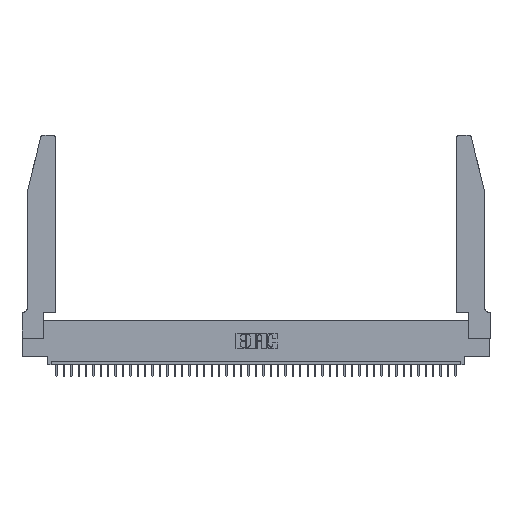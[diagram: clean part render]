
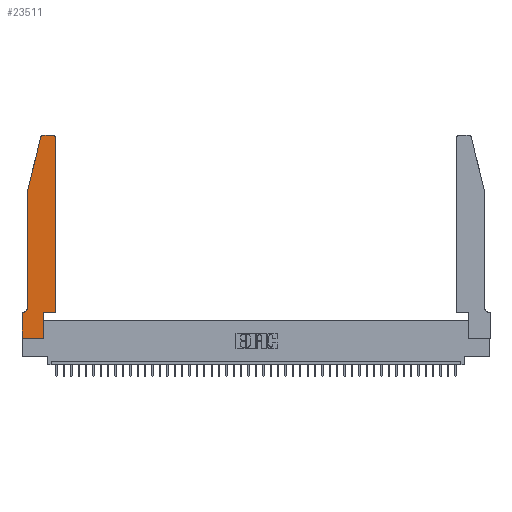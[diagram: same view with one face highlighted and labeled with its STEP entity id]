
A CAD part, top view. The second image highlights one B-rep face of the part: STEP entity #23511.
In plain terms, the highlighted planar face has unit normal (0, 0, 1).
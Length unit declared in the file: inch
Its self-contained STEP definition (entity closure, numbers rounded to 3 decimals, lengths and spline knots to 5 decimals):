
#9 = LINE ( 'NONE', #19868, #17234 ) ;
#221 = EDGE_CURVE ( 'NONE', #9567, #36295, #20676, .T. ) ;
#1085 = CIRCLE ( 'NONE', #24405, 0.07 ) ;
#1886 = DIRECTION ( 'NONE',  ( 0., 1., 0. ) ) ;
#2958 = VECTOR ( 'NONE', #28050, 39.37008 ) ;
#3400 = LINE ( 'NONE', #31642, #19021 ) ;
#4029 = CARTESIAN_POINT ( 'NONE',  ( 0.0755, 2., 0.37 ) ) ;
#4107 = EDGE_LOOP ( 'NONE', ( #40600, #10642, #42172, #23127, #11928, #31680, #28191, #36041, #9734, #17032, #40206, #28281 ) ) ;
#4935 = DIRECTION ( 'NONE',  ( -1., 0., 0. ) ) ;
#5293 = VERTEX_POINT ( 'NONE', #27888 ) ;
#7151 = DIRECTION ( 'NONE',  ( 0., 0., 1. ) ) ;
#7639 = LINE ( 'NONE', #30209, #44311 ) ;
#9567 = VERTEX_POINT ( 'NONE', #40559 ) ;
#9646 = EDGE_CURVE ( 'NONE', #19961, #39414, #7639, .T. ) ;
#9734 = ORIENTED_EDGE ( 'NONE', *, *, #16842, .T. ) ;
#10638 = CARTESIAN_POINT ( 'NONE',  ( 0.2865, 0., 0.37 ) ) ;
#10642 = ORIENTED_EDGE ( 'NONE', *, *, #14025, .T. ) ;
#10894 = EDGE_CURVE ( 'NONE', #28422, #9567, #1085, .T. ) ;
#11406 = FACE_OUTER_BOUND ( 'NONE', #4107, .T. ) ;
#11442 = DIRECTION ( 'NONE',  ( 1., 0., 0. ) ) ;
#11928 = ORIENTED_EDGE ( 'NONE', *, *, #10894, .T. ) ;
#11973 = EDGE_CURVE ( 'NONE', #24701, #5293, #9, .T. ) ;
#12093 = LINE ( 'NONE', #4029, #2958 ) ;
#12349 = LINE ( 'NONE', #12561, #28568 ) ;
#12561 = CARTESIAN_POINT ( 'NONE',  ( 0.2865, 0.35, 0.37 ) ) ;
#12959 = CARTESIAN_POINT ( 'NONE',  ( 0., 0., 0.37 ) ) ;
#13443 = VERTEX_POINT ( 'NONE', #16034 ) ;
#14023 = AXIS2_PLACEMENT_3D ( 'NONE', #44610, #16250, #37972 ) ;
#14025 = EDGE_CURVE ( 'NONE', #13443, #28636, #24495, .T. ) ;
#14664 = VECTOR ( 'NONE', #24942, 39.37008 ) ;
#15070 = CARTESIAN_POINT ( 'NONE',  ( 0.0755, 0.35, 0.37 ) ) ;
#16034 = CARTESIAN_POINT ( 'NONE',  ( 0.284, 2.75, 0.37 ) ) ;
#16250 = DIRECTION ( 'NONE',  ( 0., 0., 1. ) ) ;
#16370 = CARTESIAN_POINT ( 'NONE',  ( 0.0055, 0.42, 0.37 ) ) ;
#16842 = EDGE_CURVE ( 'NONE', #39414, #24701, #12349, .T. ) ;
#17032 = ORIENTED_EDGE ( 'NONE', *, *, #11973, .T. ) ;
#17118 = EDGE_CURVE ( 'NONE', #5293, #40108, #32338, .T. ) ;
#17234 = VECTOR ( 'NONE', #30311, 39.37008 ) ;
#17443 = VECTOR ( 'NONE', #4935, 39.37008 ) ;
#18944 = CARTESIAN_POINT ( 'NONE',  ( 0.0755, 2., 0.37 ) ) ;
#19010 = DIRECTION ( 'NONE',  ( 0., -1., 0. ) ) ;
#19021 = VECTOR ( 'NONE', #34982, 39.37008 ) ;
#19833 = CARTESIAN_POINT ( 'NONE',  ( 0.4205, 2.72, 0.37 ) ) ;
#19868 = CARTESIAN_POINT ( 'NONE',  ( 0.4505, 0.35, 0.37 ) ) ;
#19961 = VERTEX_POINT ( 'NONE', #12959 ) ;
#20088 = EDGE_CURVE ( 'NONE', #36295, #19961, #36574, .T. ) ;
#20461 = AXIS2_PLACEMENT_3D ( 'NONE', #31843, #25239, #11442 ) ;
#20675 = AXIS2_PLACEMENT_3D ( 'NONE', #19833, #7151, #38173 ) ;
#20676 = LINE ( 'NONE', #15070, #14664 ) ;
#21713 = EDGE_CURVE ( 'NONE', #28636, #37659, #12093, .T. ) ;
#21863 = EDGE_CURVE ( 'NONE', #38282, #13443, #33699, .T. ) ;
#23127 = ORIENTED_EDGE ( 'NONE', *, *, #23548, .T. ) ;
#23511 = ADVANCED_FACE ( 'NONE', ( #11406 ), #37441, .T. ) ;
#23548 = EDGE_CURVE ( 'NONE', #37659, #28422, #3400, .T. ) ;
#23856 = DIRECTION ( 'NONE',  ( 1., 0., 0. ) ) ;
#24405 = AXIS2_PLACEMENT_3D ( 'NONE', #16370, #40501, #26411 ) ;
#24495 = CIRCLE ( 'NONE', #20461, 0.03 ) ;
#24701 = VERTEX_POINT ( 'NONE', #32759 ) ;
#24942 = DIRECTION ( 'NONE',  ( -1., 0., 0. ) ) ;
#25239 = DIRECTION ( 'NONE',  ( 0., 0., 1. ) ) ;
#25637 = CARTESIAN_POINT ( 'NONE',  ( 0.2605, 2.75, 0.37 ) ) ;
#25870 = CARTESIAN_POINT ( 'NONE',  ( 0.4205, 2.75, 0.37 ) ) ;
#26411 = DIRECTION ( 'NONE',  ( -1., 0., 0. ) ) ;
#27357 = CARTESIAN_POINT ( 'NONE',  ( 0.25487, 2.72718, 0.37 ) ) ;
#27888 = CARTESIAN_POINT ( 'NONE',  ( 0.4505, 0.35, 0.37 ) ) ;
#28050 = DIRECTION ( 'NONE',  ( -0.239, -0.971, 0. ) ) ;
#28191 = ORIENTED_EDGE ( 'NONE', *, *, #20088, .T. ) ;
#28243 = CARTESIAN_POINT ( 'NONE',  ( 0., 0., 0.37 ) ) ;
#28281 = ORIENTED_EDGE ( 'NONE', *, *, #41754, .T. ) ;
#28422 = VERTEX_POINT ( 'NONE', #40388 ) ;
#28568 = VECTOR ( 'NONE', #37535, 39.37008 ) ;
#28636 = VERTEX_POINT ( 'NONE', #27357 ) ;
#30209 = CARTESIAN_POINT ( 'NONE',  ( 0., 0., 0.37 ) ) ;
#30311 = DIRECTION ( 'NONE',  ( 1., 0., 0. ) ) ;
#31642 = CARTESIAN_POINT ( 'NONE',  ( 0.0755, 2., 0.37 ) ) ;
#31680 = ORIENTED_EDGE ( 'NONE', *, *, #221, .T. ) ;
#31843 = CARTESIAN_POINT ( 'NONE',  ( 0.284, 2.72, 0.37 ) ) ;
#32338 = LINE ( 'NONE', #34852, #35027 ) ;
#32759 = CARTESIAN_POINT ( 'NONE',  ( 0.2865, 0.35, 0.37 ) ) ;
#33699 = LINE ( 'NONE', #25637, #17443 ) ;
#34852 = CARTESIAN_POINT ( 'NONE',  ( 0.4505, 0.35, 0.37 ) ) ;
#34982 = DIRECTION ( 'NONE',  ( 0., -1., 0. ) ) ;
#35027 = VECTOR ( 'NONE', #1886, 39.37008 ) ;
#36041 = ORIENTED_EDGE ( 'NONE', *, *, #9646, .T. ) ;
#36295 = VERTEX_POINT ( 'NONE', #36422 ) ;
#36422 = CARTESIAN_POINT ( 'NONE',  ( 0., 0.35, 0.37 ) ) ;
#36574 = LINE ( 'NONE', #28243, #42958 ) ;
#36603 = CIRCLE ( 'NONE', #20675, 0.03 ) ;
#37441 = PLANE ( 'NONE',  #14023 ) ;
#37535 = DIRECTION ( 'NONE',  ( 0., 1., 0. ) ) ;
#37659 = VERTEX_POINT ( 'NONE', #18944 ) ;
#37972 = DIRECTION ( 'NONE',  ( 1., 0., 0. ) ) ;
#38162 = CARTESIAN_POINT ( 'NONE',  ( 0.4505, 2.72, 0.37 ) ) ;
#38173 = DIRECTION ( 'NONE',  ( 1., 0., 0. ) ) ;
#38282 = VERTEX_POINT ( 'NONE', #25870 ) ;
#39414 = VERTEX_POINT ( 'NONE', #10638 ) ;
#40108 = VERTEX_POINT ( 'NONE', #38162 ) ;
#40206 = ORIENTED_EDGE ( 'NONE', *, *, #17118, .T. ) ;
#40388 = CARTESIAN_POINT ( 'NONE',  ( 0.0755, 0.42, 0.37 ) ) ;
#40501 = DIRECTION ( 'NONE',  ( 0., 0., -1. ) ) ;
#40559 = CARTESIAN_POINT ( 'NONE',  ( 0.0055, 0.35, 0.37 ) ) ;
#40600 = ORIENTED_EDGE ( 'NONE', *, *, #21863, .T. ) ;
#41754 = EDGE_CURVE ( 'NONE', #40108, #38282, #36603, .T. ) ;
#42172 = ORIENTED_EDGE ( 'NONE', *, *, #21713, .T. ) ;
#42958 = VECTOR ( 'NONE', #19010, 39.37008 ) ;
#44311 = VECTOR ( 'NONE', #23856, 39.37008 ) ;
#44610 = CARTESIAN_POINT ( 'NONE',  ( 0., 0.35, 0.37 ) ) ;
